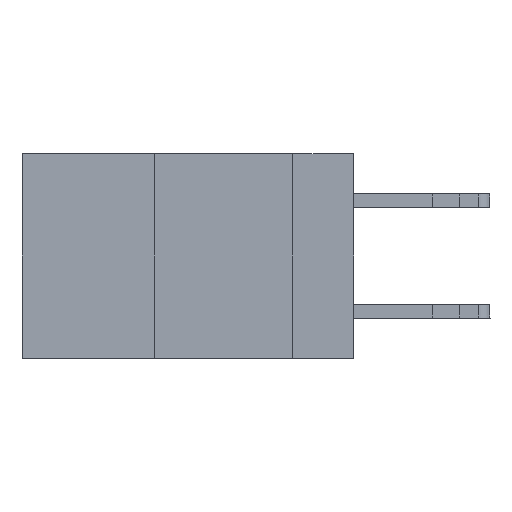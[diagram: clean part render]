
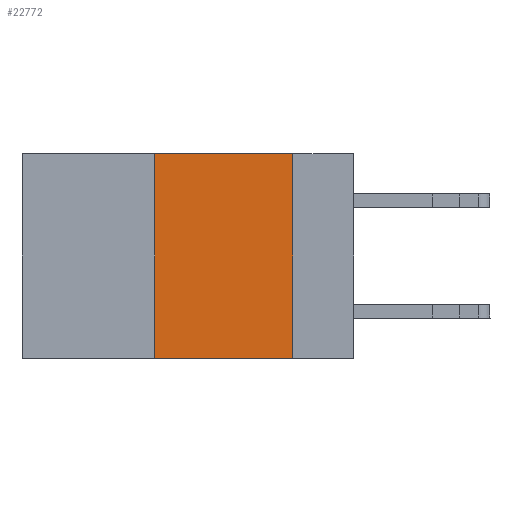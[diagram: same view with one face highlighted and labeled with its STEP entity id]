
A CAD part, left-side view. The second image highlights one B-rep face of the part: STEP entity #22772.
In plain terms, the highlighted planar face has unit normal (-1, 0, 0).
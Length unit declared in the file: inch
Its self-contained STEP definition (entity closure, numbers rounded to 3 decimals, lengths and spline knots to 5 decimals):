
#692 = CARTESIAN_POINT ( 'NONE',  ( 0., 0.36, -0.37 ) ) ;
#2504 = FACE_OUTER_BOUND ( 'NONE', #23633, .T. ) ;
#2947 = CARTESIAN_POINT ( 'NONE',  ( 0., 0.6, 0. ) ) ;
#3069 = LINE ( 'NONE', #2947, #6778 ) ;
#3329 = ORIENTED_EDGE ( 'NONE', *, *, #23815, .F. ) ;
#4507 = VERTEX_POINT ( 'NONE', #18235 ) ;
#4698 = DIRECTION ( 'NONE',  ( 0., -1., 0. ) ) ;
#5220 = VECTOR ( 'NONE', #13052, 39.37008 ) ;
#5759 = VECTOR ( 'NONE', #7324, 39.37008 ) ;
#6489 = ORIENTED_EDGE ( 'NONE', *, *, #8120, .F. ) ;
#6778 = VECTOR ( 'NONE', #4698, 39.37008 ) ;
#7324 = DIRECTION ( 'NONE',  ( 0., 0., 1. ) ) ;
#7532 = AXIS2_PLACEMENT_3D ( 'NONE', #13979, #15716, #13848 ) ;
#8120 = EDGE_CURVE ( 'NONE', #8721, #20233, #11528, .T. ) ;
#8721 = VERTEX_POINT ( 'NONE', #692 ) ;
#8735 = CARTESIAN_POINT ( 'NONE',  ( 0., 0.36, 0. ) ) ;
#9195 = CARTESIAN_POINT ( 'NONE',  ( 0., 0.11, 0. ) ) ;
#10231 = PLANE ( 'NONE',  #7532 ) ;
#10335 = EDGE_CURVE ( 'NONE', #4507, #17822, #17167, .T. ) ;
#11528 = LINE ( 'NONE', #22861, #5759 ) ;
#13052 = DIRECTION ( 'NONE',  ( 0., 0., -1. ) ) ;
#13088 = EDGE_CURVE ( 'NONE', #8721, #17822, #16346, .T. ) ;
#13848 = DIRECTION ( 'NONE',  ( 0., 0., -1. ) ) ;
#13979 = CARTESIAN_POINT ( 'NONE',  ( 0., 0.6, 0. ) ) ;
#14747 = CARTESIAN_POINT ( 'NONE',  ( 0., 0.11, -0.37 ) ) ;
#15716 = DIRECTION ( 'NONE',  ( 1., 0., 0. ) ) ;
#16346 = LINE ( 'NONE', #22046, #23193 ) ;
#17167 = LINE ( 'NONE', #9195, #5220 ) ;
#17763 = ORIENTED_EDGE ( 'NONE', *, *, #13088, .T. ) ;
#17822 = VERTEX_POINT ( 'NONE', #14747 ) ;
#18235 = CARTESIAN_POINT ( 'NONE',  ( 0., 0.11, 0. ) ) ;
#19150 = ORIENTED_EDGE ( 'NONE', *, *, #10335, .F. ) ;
#19692 = DIRECTION ( 'NONE',  ( 0., -1., 0. ) ) ;
#20233 = VERTEX_POINT ( 'NONE', #8735 ) ;
#22046 = CARTESIAN_POINT ( 'NONE',  ( 0., 0.6, -0.37 ) ) ;
#22772 = ADVANCED_FACE ( 'NONE', ( #2504 ), #10231, .F. ) ;
#22861 = CARTESIAN_POINT ( 'NONE',  ( 0., 0.36, 0. ) ) ;
#23193 = VECTOR ( 'NONE', #19692, 39.37008 ) ;
#23633 = EDGE_LOOP ( 'NONE', ( #19150, #3329, #6489, #17763 ) ) ;
#23815 = EDGE_CURVE ( 'NONE', #20233, #4507, #3069, .T. ) ;
